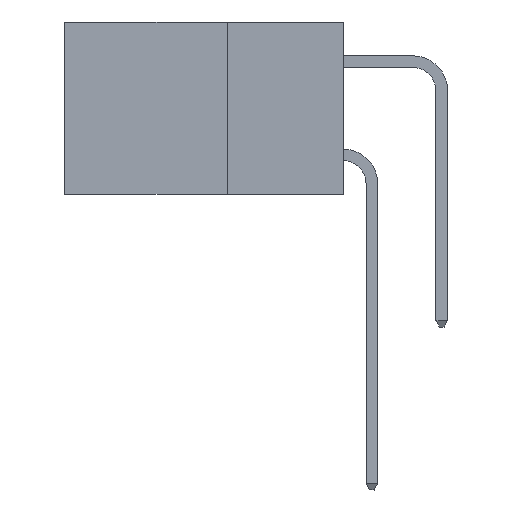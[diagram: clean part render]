
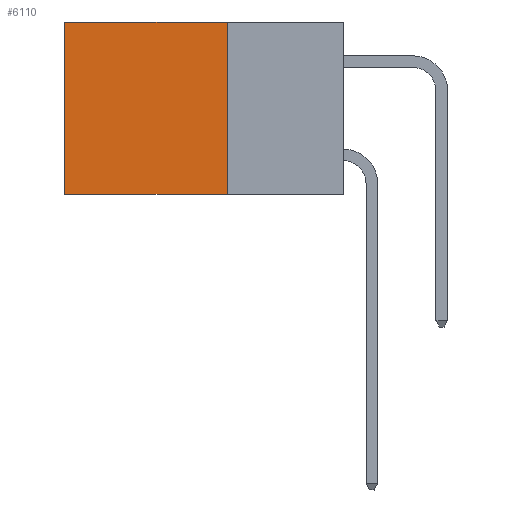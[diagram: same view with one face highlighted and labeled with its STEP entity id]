
A CAD part, left-side view. The second image highlights one B-rep face of the part: STEP entity #6110.
In plain terms, the highlighted planar face has unit normal (-1, 0, 0).
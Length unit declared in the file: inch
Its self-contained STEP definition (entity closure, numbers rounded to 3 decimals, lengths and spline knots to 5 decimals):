
#114 = VECTOR ( 'NONE', #23022, 39.37008 ) ;
#501 = CARTESIAN_POINT ( 'NONE',  ( 0.298, 0.25, 0. ) ) ;
#724 = LINE ( 'NONE', #15048, #5637 ) ;
#1363 = CARTESIAN_POINT ( 'NONE',  ( 0.298, 0.25, -0.37 ) ) ;
#1690 = EDGE_CURVE ( 'NONE', #21590, #14837, #724, .T. ) ;
#2383 = DIRECTION ( 'NONE',  ( 0., 0., -1. ) ) ;
#4507 = VECTOR ( 'NONE', #6534, 39.37008 ) ;
#4668 = EDGE_LOOP ( 'NONE', ( #7536, #5709, #11140, #19675 ) ) ;
#5637 = VECTOR ( 'NONE', #14091, 39.37008 ) ;
#5709 = ORIENTED_EDGE ( 'NONE', *, *, #1690, .F. ) ;
#5722 = VERTEX_POINT ( 'NONE', #12536 ) ;
#6110 = ADVANCED_FACE ( 'NONE', ( #20035 ), #17125, .F. ) ;
#6163 = LINE ( 'NONE', #12403, #114 ) ;
#6383 = DIRECTION ( 'NONE',  ( 1., 0., 0. ) ) ;
#6534 = DIRECTION ( 'NONE',  ( 0., 0., -1. ) ) ;
#7536 = ORIENTED_EDGE ( 'NONE', *, *, #20803, .T. ) ;
#8734 = LINE ( 'NONE', #17273, #4507 ) ;
#10601 = CARTESIAN_POINT ( 'NONE',  ( 0.298, 0.6, -0.37 ) ) ;
#11140 = ORIENTED_EDGE ( 'NONE', *, *, #12355, .F. ) ;
#11682 = VECTOR ( 'NONE', #2383, 39.37008 ) ;
#12355 = EDGE_CURVE ( 'NONE', #5722, #21590, #21158, .T. ) ;
#12403 = CARTESIAN_POINT ( 'NONE',  ( 0.298, 0.25, 0. ) ) ;
#12536 = CARTESIAN_POINT ( 'NONE',  ( 0.298, 0.25, 0. ) ) ;
#14091 = DIRECTION ( 'NONE',  ( 0., 1., 0. ) ) ;
#14365 = VERTEX_POINT ( 'NONE', #18295 ) ;
#14837 = VERTEX_POINT ( 'NONE', #10601 ) ;
#15048 = CARTESIAN_POINT ( 'NONE',  ( 0.298, 0.25, -0.37 ) ) ;
#16226 = EDGE_CURVE ( 'NONE', #5722, #14365, #6163, .T. ) ;
#17125 = PLANE ( 'NONE',  #19378 ) ;
#17273 = CARTESIAN_POINT ( 'NONE',  ( 0.298, 0.6, 0. ) ) ;
#18295 = CARTESIAN_POINT ( 'NONE',  ( 0.298, 0.6, 0. ) ) ;
#18846 = CARTESIAN_POINT ( 'NONE',  ( 0.298, 0.25, 0. ) ) ;
#18928 = DIRECTION ( 'NONE',  ( 0., 0., -1. ) ) ;
#19378 = AXIS2_PLACEMENT_3D ( 'NONE', #18846, #6383, #18928 ) ;
#19675 = ORIENTED_EDGE ( 'NONE', *, *, #16226, .T. ) ;
#20035 = FACE_OUTER_BOUND ( 'NONE', #4668, .T. ) ;
#20803 = EDGE_CURVE ( 'NONE', #14365, #14837, #8734, .T. ) ;
#21158 = LINE ( 'NONE', #501, #11682 ) ;
#21590 = VERTEX_POINT ( 'NONE', #1363 ) ;
#23022 = DIRECTION ( 'NONE',  ( 0., 1., 0. ) ) ;
